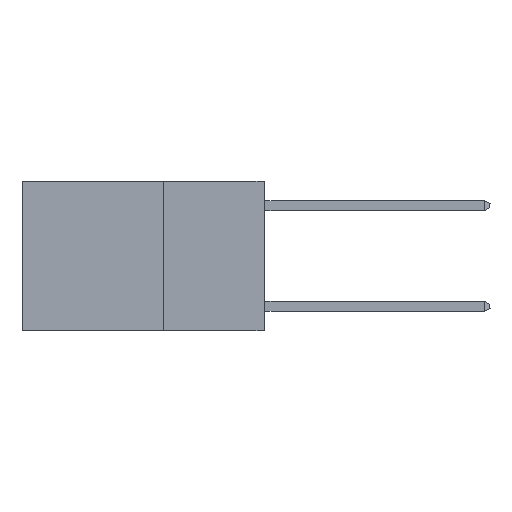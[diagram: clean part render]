
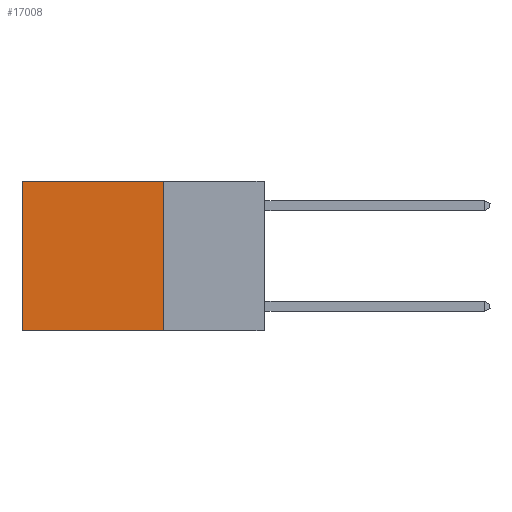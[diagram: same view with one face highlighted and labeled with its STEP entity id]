
A CAD part, left-side view. The second image highlights one B-rep face of the part: STEP entity #17008.
In plain terms, the highlighted planar face has unit normal (-1, 0, 0).
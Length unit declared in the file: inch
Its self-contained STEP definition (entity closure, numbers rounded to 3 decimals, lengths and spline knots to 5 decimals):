
#619 = LINE ( 'NONE', #8573, #14295 ) ;
#1483 = EDGE_LOOP ( 'NONE', ( #15972, #24821, #4578, #15762 ) ) ;
#4192 = AXIS2_PLACEMENT_3D ( 'NONE', #11408, #11013, #7466 ) ;
#4578 = ORIENTED_EDGE ( 'NONE', *, *, #22987, .F. ) ;
#4768 = EDGE_CURVE ( 'NONE', #19255, #15923, #13371, .T. ) ;
#4835 = VECTOR ( 'NONE', #16904, 39.37008 ) ;
#4958 = LINE ( 'NONE', #21480, #23118 ) ;
#5877 = EDGE_CURVE ( 'NONE', #25454, #15923, #13316, .T. ) ;
#5886 = DIRECTION ( 'NONE',  ( 0., 1., 0. ) ) ;
#7338 = FACE_OUTER_BOUND ( 'NONE', #1483, .T. ) ;
#7466 = DIRECTION ( 'NONE',  ( 0., 0., -1. ) ) ;
#8573 = CARTESIAN_POINT ( 'NONE',  ( 0.2625, 0.25, 0. ) ) ;
#9460 = CARTESIAN_POINT ( 'NONE',  ( 0.2625, 0.25, -0.37 ) ) ;
#10286 = DIRECTION ( 'NONE',  ( 0., 0., -1. ) ) ;
#11013 = DIRECTION ( 'NONE',  ( 1., 0., 0. ) ) ;
#11408 = CARTESIAN_POINT ( 'NONE',  ( 0.2625, 0.25, 0. ) ) ;
#13102 = VECTOR ( 'NONE', #15400, 39.37008 ) ;
#13316 = LINE ( 'NONE', #21105, #4835 ) ;
#13371 = LINE ( 'NONE', #21569, #13102 ) ;
#14295 = VECTOR ( 'NONE', #10286, 39.37008 ) ;
#14626 = EDGE_CURVE ( 'NONE', #17171, #25454, #4958, .T. ) ;
#15400 = DIRECTION ( 'NONE',  ( 0., 1., 0. ) ) ;
#15762 = ORIENTED_EDGE ( 'NONE', *, *, #14626, .T. ) ;
#15923 = VERTEX_POINT ( 'NONE', #22761 ) ;
#15972 = ORIENTED_EDGE ( 'NONE', *, *, #5877, .T. ) ;
#16904 = DIRECTION ( 'NONE',  ( 0., 0., -1. ) ) ;
#17008 = ADVANCED_FACE ( 'NONE', ( #7338 ), #19572, .F. ) ;
#17171 = VERTEX_POINT ( 'NONE', #22508 ) ;
#19255 = VERTEX_POINT ( 'NONE', #9460 ) ;
#19572 = PLANE ( 'NONE',  #4192 ) ;
#19816 = CARTESIAN_POINT ( 'NONE',  ( 0.2625, 0.6, 0. ) ) ;
#21105 = CARTESIAN_POINT ( 'NONE',  ( 0.2625, 0.6, 0. ) ) ;
#21480 = CARTESIAN_POINT ( 'NONE',  ( 0.2625, 0.25, 0. ) ) ;
#21569 = CARTESIAN_POINT ( 'NONE',  ( 0.2625, 0.25, -0.37 ) ) ;
#22508 = CARTESIAN_POINT ( 'NONE',  ( 0.2625, 0.25, 0. ) ) ;
#22761 = CARTESIAN_POINT ( 'NONE',  ( 0.2625, 0.6, -0.37 ) ) ;
#22987 = EDGE_CURVE ( 'NONE', #17171, #19255, #619, .T. ) ;
#23118 = VECTOR ( 'NONE', #5886, 39.37008 ) ;
#24821 = ORIENTED_EDGE ( 'NONE', *, *, #4768, .F. ) ;
#25454 = VERTEX_POINT ( 'NONE', #19816 ) ;
